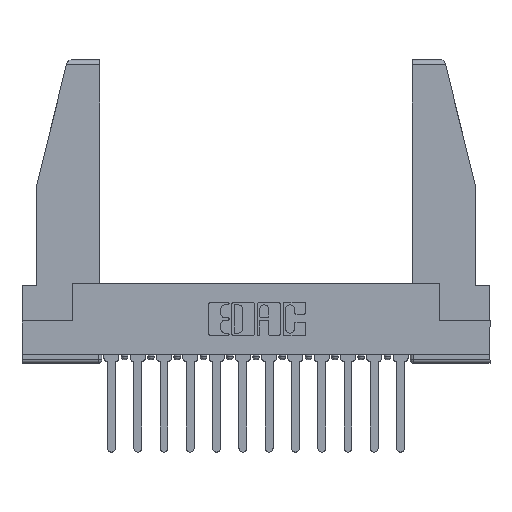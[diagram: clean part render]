
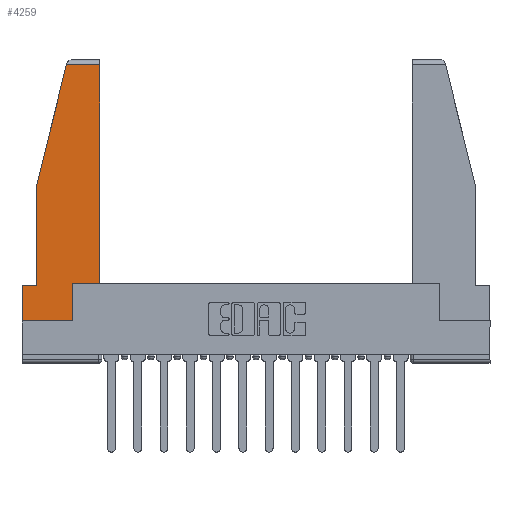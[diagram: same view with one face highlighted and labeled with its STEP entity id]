
A CAD part, top view. The second image highlights one B-rep face of the part: STEP entity #4259.
In plain terms, the highlighted planar face has unit normal (0, 0, 1).
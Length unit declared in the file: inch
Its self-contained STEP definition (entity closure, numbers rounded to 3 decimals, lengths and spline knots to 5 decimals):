
#65 = CARTESIAN_POINT ( 'NONE',  ( 0.297, 0., 0. ) ) ;
#92 = VERTEX_POINT ( 'NONE', #4076 ) ;
#589 = VECTOR ( 'NONE', #8007, 39.37008 ) ;
#742 = EDGE_CURVE ( 'NONE', #12525, #16297, #8583, .T. ) ;
#794 = VERTEX_POINT ( 'NONE', #16073 ) ;
#825 = EDGE_CURVE ( 'NONE', #92, #10112, #14710, .T. ) ;
#845 = CARTESIAN_POINT ( 'NONE',  ( 0.461, 0.223, 0. ) ) ;
#1245 = CARTESIAN_POINT ( 'NONE',  ( 0.086, 0.8, 0. ) ) ;
#1782 = VECTOR ( 'NONE', #6814, 39.37008 ) ;
#1992 = DIRECTION ( 'NONE',  ( 0., -1., 0. ) ) ;
#2604 = DIRECTION ( 'NONE',  ( -1., 0., 0. ) ) ;
#2733 = ORIENTED_EDGE ( 'NONE', *, *, #9659, .T. ) ;
#2734 = CARTESIAN_POINT ( 'NONE',  ( 0.297, 0., 0. ) ) ;
#2965 = ORIENTED_EDGE ( 'NONE', *, *, #6819, .T. ) ;
#3057 = CARTESIAN_POINT ( 'NONE',  ( 0.297, 0.223, 0. ) ) ;
#3108 = PLANE ( 'NONE',  #13538 ) ;
#4076 = CARTESIAN_POINT ( 'NONE',  ( 0.297, 0.223, 0. ) ) ;
#4259 = ADVANCED_FACE ( 'NONE', ( #11013 ), #3108, .T. ) ;
#4686 = CARTESIAN_POINT ( 'NONE',  ( 0., 0., 0. ) ) ;
#5297 = VERTEX_POINT ( 'NONE', #15722 ) ;
#5374 = LINE ( 'NONE', #15748, #589 ) ;
#5652 = EDGE_CURVE ( 'NONE', #794, #12525, #16790, .T. ) ;
#5994 = EDGE_CURVE ( 'NONE', #10112, #8052, #5374, .T. ) ;
#6320 = VECTOR ( 'NONE', #2604, 39.37008 ) ;
#6814 = DIRECTION ( 'NONE',  ( 0., 1., 0. ) ) ;
#6819 = EDGE_CURVE ( 'NONE', #16297, #5297, #16641, .T. ) ;
#8007 = DIRECTION ( 'NONE',  ( 0., 1., 0. ) ) ;
#8052 = VERTEX_POINT ( 'NONE', #8821 ) ;
#8250 = DIRECTION ( 'NONE',  ( 1., 0., 0. ) ) ;
#8583 = LINE ( 'NONE', #12324, #16081 ) ;
#8747 = VECTOR ( 'NONE', #8250, 39.37008 ) ;
#8821 = CARTESIAN_POINT ( 'NONE',  ( 0.461, 1.52, 0. ) ) ;
#9071 = CARTESIAN_POINT ( 'NONE',  ( 0., 0.21, 0. ) ) ;
#9659 = EDGE_CURVE ( 'NONE', #5297, #11153, #16360, .T. ) ;
#9788 = EDGE_LOOP ( 'NONE', ( #12002, #11000, #14242, #13554, #2965, #2733, #16171, #15608, #15420 ) ) ;
#9902 = EDGE_CURVE ( 'NONE', #15213, #92, #14386, .T. ) ;
#10112 = VERTEX_POINT ( 'NONE', #845 ) ;
#10326 = CARTESIAN_POINT ( 'NONE',  ( 0.271, 1.55, 0. ) ) ;
#10330 = CARTESIAN_POINT ( 'NONE',  ( 0., 0., 0. ) ) ;
#10521 = VECTOR ( 'NONE', #13603, 39.37008 ) ;
#10622 = LINE ( 'NONE', #13255, #15871 ) ;
#10857 = DIRECTION ( 'NONE',  ( 0., 0., 1. ) ) ;
#11000 = ORIENTED_EDGE ( 'NONE', *, *, #16597, .T. ) ;
#11013 = FACE_OUTER_BOUND ( 'NONE', #9788, .T. ) ;
#11138 = DIRECTION ( 'NONE',  ( 0., -1., 0. ) ) ;
#11153 = VERTEX_POINT ( 'NONE', #10330 ) ;
#12002 = ORIENTED_EDGE ( 'NONE', *, *, #5994, .T. ) ;
#12324 = CARTESIAN_POINT ( 'NONE',  ( 0.086, 0.8, 0. ) ) ;
#12525 = VERTEX_POINT ( 'NONE', #1245 ) ;
#13169 = DIRECTION ( 'NONE',  ( -1., 0., 0. ) ) ;
#13200 = EDGE_CURVE ( 'NONE', #11153, #15213, #16082, .T. ) ;
#13255 = CARTESIAN_POINT ( 'NONE',  ( 0., 1.52, 0. ) ) ;
#13538 = AXIS2_PLACEMENT_3D ( 'NONE', #13646, #10857, #16046 ) ;
#13554 = ORIENTED_EDGE ( 'NONE', *, *, #742, .T. ) ;
#13603 = DIRECTION ( 'NONE',  ( 1., 0., 0. ) ) ;
#13646 = CARTESIAN_POINT ( 'NONE',  ( 0., 0., 0. ) ) ;
#14242 = ORIENTED_EDGE ( 'NONE', *, *, #5652, .T. ) ;
#14386 = LINE ( 'NONE', #2734, #1782 ) ;
#14710 = LINE ( 'NONE', #3057, #8747 ) ;
#14952 = CARTESIAN_POINT ( 'NONE',  ( 0.086, 0.21, 0. ) ) ;
#15089 = CARTESIAN_POINT ( 'NONE',  ( 0., 0.21, 0. ) ) ;
#15213 = VERTEX_POINT ( 'NONE', #65 ) ;
#15420 = ORIENTED_EDGE ( 'NONE', *, *, #825, .T. ) ;
#15515 = DIRECTION ( 'NONE',  ( -0.239, -0.971, 0. ) ) ;
#15608 = ORIENTED_EDGE ( 'NONE', *, *, #9902, .T. ) ;
#15623 = VECTOR ( 'NONE', #1992, 39.37008 ) ;
#15722 = CARTESIAN_POINT ( 'NONE',  ( 0., 0.21, 0. ) ) ;
#15748 = CARTESIAN_POINT ( 'NONE',  ( 0.461, 0.223, 0. ) ) ;
#15871 = VECTOR ( 'NONE', #13169, 39.37008 ) ;
#16046 = DIRECTION ( 'NONE',  ( 1., 0., 0. ) ) ;
#16073 = CARTESIAN_POINT ( 'NONE',  ( 0.2636, 1.52, 0. ) ) ;
#16081 = VECTOR ( 'NONE', #11138, 39.37008 ) ;
#16082 = LINE ( 'NONE', #4686, #10521 ) ;
#16171 = ORIENTED_EDGE ( 'NONE', *, *, #13200, .T. ) ;
#16297 = VERTEX_POINT ( 'NONE', #14952 ) ;
#16326 = VECTOR ( 'NONE', #15515, 39.37008 ) ;
#16360 = LINE ( 'NONE', #15089, #15623 ) ;
#16597 = EDGE_CURVE ( 'NONE', #8052, #794, #10622, .T. ) ;
#16641 = LINE ( 'NONE', #9071, #6320 ) ;
#16790 = LINE ( 'NONE', #10326, #16326 ) ;
